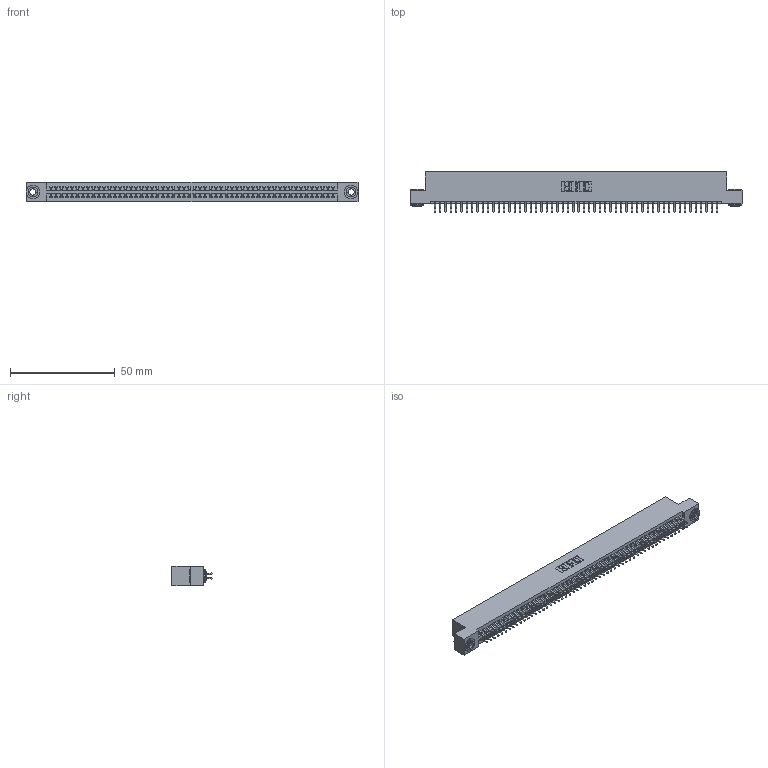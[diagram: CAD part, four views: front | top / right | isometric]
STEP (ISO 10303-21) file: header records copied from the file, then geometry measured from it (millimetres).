
FILE_DESCRIPTION (( 'STEP AP203' ), '1' );
FILE_NAME ('395-108-556-203.STEP', '2018-11-30T23:27:17', ( '' ), ( '' ), 'SwSTEP 2.0', 'SolidWorks 2016', '' );
FILE_SCHEMA (( 'CONFIG_CONTROL_DESIGN' ));
Length unit declared in the file: inch
Products named in the file (4): 395-108-556-203; 345 Part_Flush Mounting Lugs - 0.156 Dia-TH; 345-292-001_556 Tail; 345-250-002_345-250-002-102
Assembly tree (111 placements, depth 2):
  395-108-556-203
    345 Part_Flush Mounting Lugs - 0.156 Dia-TH
    345-292-001_556 Tail  x108
    345-250-002_345-250-002-102  x2
Bounding box: 158.37 x 19.24 x 9.4 mm (x, y, z)
Volume: 15510.6 mm3; surface area: 23270.1 mm2
Topology: 111 solids, 111 shells, 6212 faces, 18453 edges, 12154 vertices
Faces by surface type: plane 4086, cylinder 2118, cone 8
Entity records: 41624 total; most frequent: CARTESIAN_POINT 6955, ORIENTED_EDGE 6870, DIRECTION 6137, EDGE_CURVE 3435, VECTOR 3055, LINE 3055, VERTEX_POINT 2286, AXIS2_PLACEMENT_3D 1541
